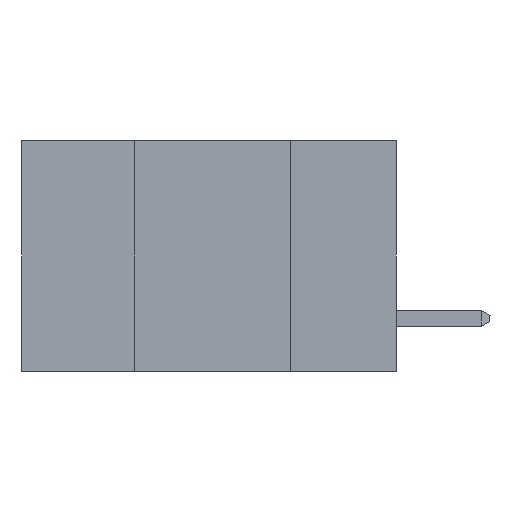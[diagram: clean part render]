
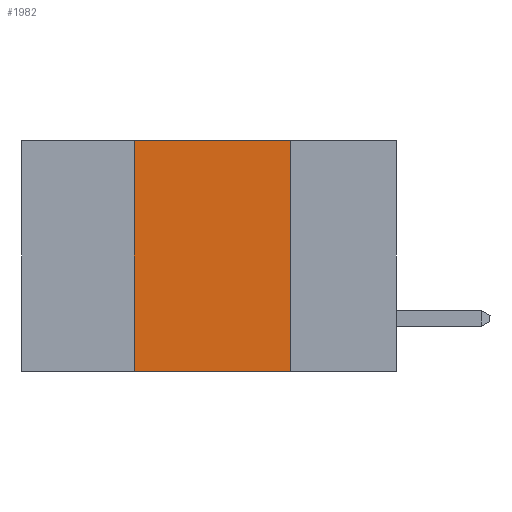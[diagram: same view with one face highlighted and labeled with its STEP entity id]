
A CAD part, left-side view. The second image highlights one B-rep face of the part: STEP entity #1982.
In plain terms, the highlighted planar face has unit normal (-1, 0, 0).
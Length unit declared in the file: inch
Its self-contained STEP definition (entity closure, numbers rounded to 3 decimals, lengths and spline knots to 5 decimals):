
#1486 = DIRECTION ( 'NONE',  ( 0., -1., 0. ) ) ;
#1790 = CARTESIAN_POINT ( 'NONE',  ( 0., 0.42, 0. ) ) ;
#1827 = EDGE_CURVE ( 'NONE', #8118, #11706, #10485, .T. ) ;
#1982 = ADVANCED_FACE ( 'NONE', ( #8272 ), #9476, .F. ) ;
#2396 = DIRECTION ( 'NONE',  ( 0., -1., 0. ) ) ;
#2485 = EDGE_CURVE ( 'NONE', #8118, #7257, #6463, .T. ) ;
#2777 = CARTESIAN_POINT ( 'NONE',  ( 0., 0.6, 0. ) ) ;
#3115 = VECTOR ( 'NONE', #13609, 39.37008 ) ;
#3738 = ORIENTED_EDGE ( 'NONE', *, *, #2485, .F. ) ;
#4331 = CARTESIAN_POINT ( 'NONE',  ( 0., 0.17, -0.37 ) ) ;
#4957 = ORIENTED_EDGE ( 'NONE', *, *, #1827, .T. ) ;
#5593 = EDGE_CURVE ( 'NONE', #7257, #8792, #11870, .T. ) ;
#5658 = CARTESIAN_POINT ( 'NONE',  ( 0., 0.17, -0.37 ) ) ;
#6111 = CARTESIAN_POINT ( 'NONE',  ( 0., 0.17, 0. ) ) ;
#6145 = DIRECTION ( 'NONE',  ( 1., 0., 0. ) ) ;
#6358 = CARTESIAN_POINT ( 'NONE',  ( 0., 0.42, -0.37 ) ) ;
#6463 = LINE ( 'NONE', #14536, #9921 ) ;
#6535 = EDGE_CURVE ( 'NONE', #8792, #11706, #10034, .T. ) ;
#6546 = DIRECTION ( 'NONE',  ( 0., 0., 1. ) ) ;
#7078 = CARTESIAN_POINT ( 'NONE',  ( 0., 0.6, -0.37 ) ) ;
#7257 = VERTEX_POINT ( 'NONE', #1790 ) ;
#7338 = AXIS2_PLACEMENT_3D ( 'NONE', #8709, #6145, #14128 ) ;
#7835 = EDGE_LOOP ( 'NONE', ( #14723, #10641, #3738, #4957 ) ) ;
#8006 = VECTOR ( 'NONE', #1486, 39.37008 ) ;
#8118 = VERTEX_POINT ( 'NONE', #6358 ) ;
#8272 = FACE_OUTER_BOUND ( 'NONE', #7835, .T. ) ;
#8709 = CARTESIAN_POINT ( 'NONE',  ( 0., 0.6, 0. ) ) ;
#8792 = VERTEX_POINT ( 'NONE', #6111 ) ;
#9476 = PLANE ( 'NONE',  #7338 ) ;
#9921 = VECTOR ( 'NONE', #6546, 39.37008 ) ;
#10034 = LINE ( 'NONE', #4331, #3115 ) ;
#10485 = LINE ( 'NONE', #7078, #11416 ) ;
#10641 = ORIENTED_EDGE ( 'NONE', *, *, #5593, .F. ) ;
#11416 = VECTOR ( 'NONE', #2396, 39.37008 ) ;
#11706 = VERTEX_POINT ( 'NONE', #5658 ) ;
#11870 = LINE ( 'NONE', #2777, #8006 ) ;
#13609 = DIRECTION ( 'NONE',  ( 0., 0., -1. ) ) ;
#14128 = DIRECTION ( 'NONE',  ( 0., 0., -1. ) ) ;
#14536 = CARTESIAN_POINT ( 'NONE',  ( 0., 0.42, -0.37 ) ) ;
#14723 = ORIENTED_EDGE ( 'NONE', *, *, #6535, .F. ) ;
